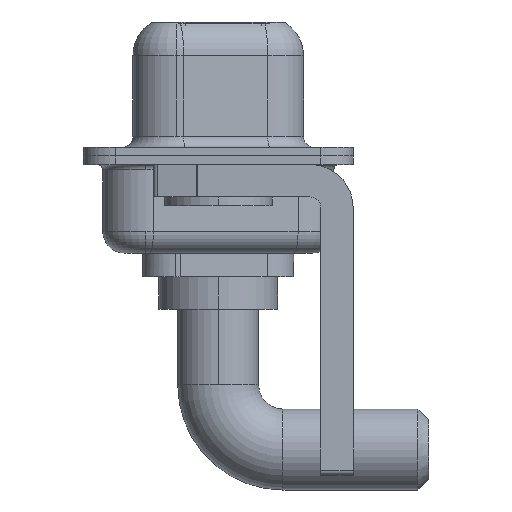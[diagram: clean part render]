
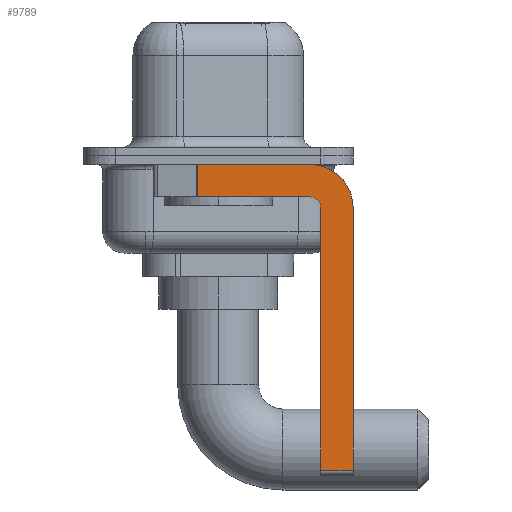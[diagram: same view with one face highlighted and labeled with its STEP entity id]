
A CAD part, left-side view. The second image highlights one B-rep face of the part: STEP entity #9789.
In plain terms, the highlighted planar face has unit normal (-1, 0, 0).
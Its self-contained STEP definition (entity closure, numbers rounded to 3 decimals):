
#87 = ORIENTED_EDGE ( 'NONE', *, *, #6880, .T. ) ;
#232 = VERTEX_POINT ( 'NONE', #5314 ) ;
#499 = VERTEX_POINT ( 'NONE', #12935 ) ;
#671 = EDGE_CURVE ( 'NONE', #5803, #4014, #9308, .T. ) ;
#1768 = CARTESIAN_POINT ( 'NONE',  ( -2.9, -4.75, -14.8 ) ) ;
#1842 = VECTOR ( 'NONE', #10129, 1000. ) ;
#1907 = ORIENTED_EDGE ( 'NONE', *, *, #6685, .T. ) ;
#2177 = DIRECTION ( 'NONE',  ( 1., 0., 0. ) ) ;
#2355 = CARTESIAN_POINT ( 'NONE',  ( -2.9, -4.25, -2.4 ) ) ;
#2688 = CARTESIAN_POINT ( 'NONE',  ( -2.9, -4.25, -1.9 ) ) ;
#3859 = VERTEX_POINT ( 'NONE', #8956 ) ;
#4012 = CARTESIAN_POINT ( 'NONE',  ( -2.9, 0.978, -1.9 ) ) ;
#4014 = VERTEX_POINT ( 'NONE', #7549 ) ;
#4120 = CARTESIAN_POINT ( 'NONE',  ( -2.9, -4.25, -0.4 ) ) ;
#4396 = LINE ( 'NONE', #8444, #12875 ) ;
#4421 = VECTOR ( 'NONE', #12988, 1000. ) ;
#4519 = CARTESIAN_POINT ( 'NONE',  ( -2.9, -4.75, -14.55 ) ) ;
#4563 = LINE ( 'NONE', #12536, #9785 ) ;
#5071 = PLANE ( 'NONE',  #6182 ) ;
#5248 = EDGE_CURVE ( 'NONE', #5469, #3859, #5672, .T. ) ;
#5274 = LINE ( 'NONE', #7003, #4421 ) ;
#5285 = CARTESIAN_POINT ( 'NONE',  ( -2.9, -6.25, -14.55 ) ) ;
#5314 = CARTESIAN_POINT ( 'NONE',  ( -2.9, 0.978, -0.4 ) ) ;
#5469 = VERTEX_POINT ( 'NONE', #5526 ) ;
#5498 = VERTEX_POINT ( 'NONE', #4519 ) ;
#5510 = AXIS2_PLACEMENT_3D ( 'NONE', #10413, #2177, #12396 ) ;
#5526 = CARTESIAN_POINT ( 'NONE',  ( -2.9, -4.25, -1.9 ) ) ;
#5672 = LINE ( 'NONE', #2688, #1842 ) ;
#5694 = CIRCLE ( 'NONE', #9079, 0.5 ) ;
#5803 = VERTEX_POINT ( 'NONE', #4120 ) ;
#5816 = DIRECTION ( 'NONE',  ( 0., 0., 1. ) ) ;
#6155 = EDGE_CURVE ( 'NONE', #5498, #499, #12853, .T. ) ;
#6168 = VERTEX_POINT ( 'NONE', #5285 ) ;
#6182 = AXIS2_PLACEMENT_3D ( 'NONE', #12898, #7840, #9236 ) ;
#6332 = DIRECTION ( 'NONE',  ( -1., 0., 0. ) ) ;
#6454 = DIRECTION ( 'NONE',  ( 0., -1., 0. ) ) ;
#6685 = EDGE_CURVE ( 'NONE', #232, #3859, #13106, .T. ) ;
#6696 = VECTOR ( 'NONE', #5816, 1000. ) ;
#6880 = EDGE_CURVE ( 'NONE', #5498, #6168, #4396, .T. ) ;
#6915 = VECTOR ( 'NONE', #11777, 1000. ) ;
#7003 = CARTESIAN_POINT ( 'NONE',  ( -2.9, 3., -0.4 ) ) ;
#7549 = CARTESIAN_POINT ( 'NONE',  ( -2.9, -6.25, -2.4 ) ) ;
#7840 = DIRECTION ( 'NONE',  ( 1., 0., 0. ) ) ;
#8053 = ORIENTED_EDGE ( 'NONE', *, *, #8170, .F. ) ;
#8170 = EDGE_CURVE ( 'NONE', #232, #5803, #5274, .T. ) ;
#8237 = EDGE_CURVE ( 'NONE', #499, #5469, #5694, .T. ) ;
#8274 = ORIENTED_EDGE ( 'NONE', *, *, #671, .F. ) ;
#8444 = CARTESIAN_POINT ( 'NONE',  ( -2.9, -4.25, -14.55 ) ) ;
#8956 = CARTESIAN_POINT ( 'NONE',  ( -2.9, 0.978, -1.9 ) ) ;
#9079 = AXIS2_PLACEMENT_3D ( 'NONE', #2355, #6332, #11011 ) ;
#9198 = EDGE_CURVE ( 'NONE', #4014, #6168, #4563, .T. ) ;
#9236 = DIRECTION ( 'NONE',  ( 0., 0., -1. ) ) ;
#9308 = CIRCLE ( 'NONE', #5510, 2. ) ;
#9785 = VECTOR ( 'NONE', #10421, 1000. ) ;
#9789 = ADVANCED_FACE ( 'NONE', ( #10049 ), #5071, .F. ) ;
#10049 = FACE_OUTER_BOUND ( 'NONE', #12900, .T. ) ;
#10129 = DIRECTION ( 'NONE',  ( 0., 1., 0. ) ) ;
#10235 = ORIENTED_EDGE ( 'NONE', *, *, #6155, .F. ) ;
#10413 = CARTESIAN_POINT ( 'NONE',  ( -2.9, -4.25, -2.4 ) ) ;
#10421 = DIRECTION ( 'NONE',  ( 0., 0., -1. ) ) ;
#11011 = DIRECTION ( 'NONE',  ( 0., 0., 1. ) ) ;
#11450 = ORIENTED_EDGE ( 'NONE', *, *, #5248, .F. ) ;
#11777 = DIRECTION ( 'NONE',  ( 0., 0., -1. ) ) ;
#12221 = ORIENTED_EDGE ( 'NONE', *, *, #9198, .F. ) ;
#12318 = ORIENTED_EDGE ( 'NONE', *, *, #8237, .F. ) ;
#12396 = DIRECTION ( 'NONE',  ( 0., 0., -1. ) ) ;
#12536 = CARTESIAN_POINT ( 'NONE',  ( -2.9, -6.25, -2.4 ) ) ;
#12853 = LINE ( 'NONE', #1768, #6696 ) ;
#12875 = VECTOR ( 'NONE', #6454, 1000. ) ;
#12898 = CARTESIAN_POINT ( 'NONE',  ( -2.9, -4.25, -2.4 ) ) ;
#12900 = EDGE_LOOP ( 'NONE', ( #8053, #1907, #11450, #12318, #10235, #87, #12221, #8274 ) ) ;
#12935 = CARTESIAN_POINT ( 'NONE',  ( -2.9, -4.75, -2.4 ) ) ;
#12988 = DIRECTION ( 'NONE',  ( 0., -1., 0. ) ) ;
#13106 = LINE ( 'NONE', #4012, #6915 ) ;
